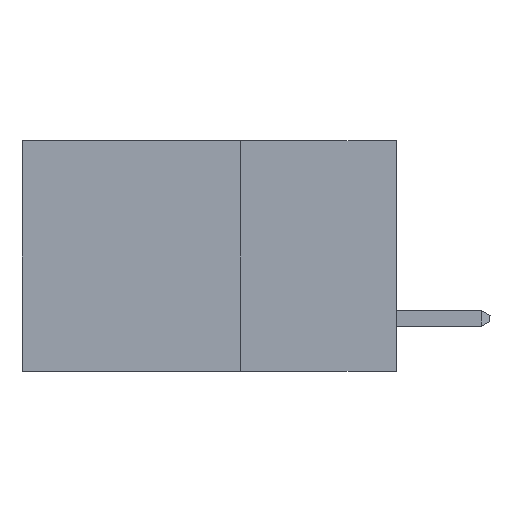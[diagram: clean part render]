
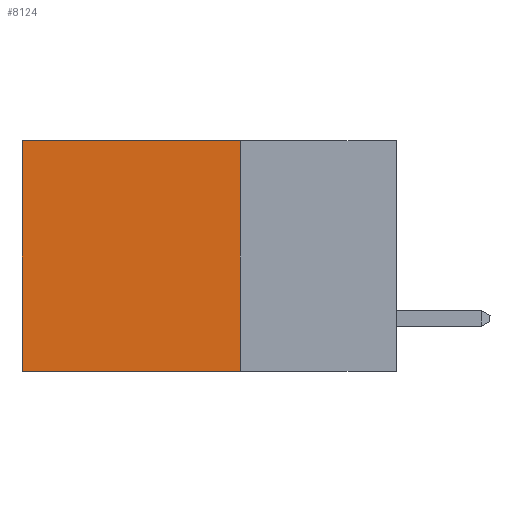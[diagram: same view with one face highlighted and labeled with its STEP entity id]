
A CAD part, left-side view. The second image highlights one B-rep face of the part: STEP entity #8124.
In plain terms, the highlighted planar face has unit normal (-1, 0, 0).
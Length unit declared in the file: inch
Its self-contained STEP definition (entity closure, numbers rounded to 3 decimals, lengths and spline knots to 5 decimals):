
#63 = VERTEX_POINT ( 'NONE', #6764 ) ;
#292 = DIRECTION ( 'NONE',  ( 0., 0., -1. ) ) ;
#690 = CARTESIAN_POINT ( 'NONE',  ( 0.2615, 0.25, -0.37 ) ) ;
#862 = VECTOR ( 'NONE', #292, 39.37008 ) ;
#1354 = CARTESIAN_POINT ( 'NONE',  ( 0.2615, 0.25, -0.37 ) ) ;
#1498 = DIRECTION ( 'NONE',  ( 0., 0., -1. ) ) ;
#1545 = FACE_OUTER_BOUND ( 'NONE', #8074, .T. ) ;
#1760 = ORIENTED_EDGE ( 'NONE', *, *, #3290, .F. ) ;
#1971 = LINE ( 'NONE', #5686, #862 ) ;
#2251 = DIRECTION ( 'NONE',  ( 1., 0., 0. ) ) ;
#2774 = EDGE_CURVE ( 'NONE', #63, #3135, #9484, .T. ) ;
#2840 = PLANE ( 'NONE',  #4221 ) ;
#3135 = VERTEX_POINT ( 'NONE', #9523 ) ;
#3290 = EDGE_CURVE ( 'NONE', #9681, #4045, #6729, .T. ) ;
#3715 = CARTESIAN_POINT ( 'NONE',  ( 0.2615, 0.6, -0.37 ) ) ;
#4045 = VERTEX_POINT ( 'NONE', #3715 ) ;
#4221 = AXIS2_PLACEMENT_3D ( 'NONE', #1354, #2251, #1498 ) ;
#4365 = VECTOR ( 'NONE', #9717, 39.37008 ) ;
#4622 = VECTOR ( 'NONE', #8279, 39.37008 ) ;
#4919 = EDGE_CURVE ( 'NONE', #3135, #4045, #1971, .T. ) ;
#5328 = LINE ( 'NONE', #8224, #4365 ) ;
#5660 = ORIENTED_EDGE ( 'NONE', *, *, #7139, .F. ) ;
#5686 = CARTESIAN_POINT ( 'NONE',  ( 0.2615, 0.6, -0.37 ) ) ;
#6640 = ORIENTED_EDGE ( 'NONE', *, *, #4919, .T. ) ;
#6729 = LINE ( 'NONE', #690, #4622 ) ;
#6764 = CARTESIAN_POINT ( 'NONE',  ( 0.2615, 0.25, 0. ) ) ;
#7139 = EDGE_CURVE ( 'NONE', #63, #9681, #5328, .T. ) ;
#7355 = CARTESIAN_POINT ( 'NONE',  ( 0.2615, 0.25, 0. ) ) ;
#7368 = VECTOR ( 'NONE', #8041, 39.37008 ) ;
#8041 = DIRECTION ( 'NONE',  ( 0., 1., 0. ) ) ;
#8074 = EDGE_LOOP ( 'NONE', ( #6640, #1760, #5660, #9621 ) ) ;
#8124 = ADVANCED_FACE ( 'NONE', ( #1545 ), #2840, .F. ) ;
#8224 = CARTESIAN_POINT ( 'NONE',  ( 0.2615, 0.25, -0.37 ) ) ;
#8253 = CARTESIAN_POINT ( 'NONE',  ( 0.2615, 0.25, -0.37 ) ) ;
#8279 = DIRECTION ( 'NONE',  ( 0., 1., 0. ) ) ;
#9484 = LINE ( 'NONE', #7355, #7368 ) ;
#9523 = CARTESIAN_POINT ( 'NONE',  ( 0.2615, 0.6, 0. ) ) ;
#9621 = ORIENTED_EDGE ( 'NONE', *, *, #2774, .T. ) ;
#9681 = VERTEX_POINT ( 'NONE', #8253 ) ;
#9717 = DIRECTION ( 'NONE',  ( 0., 0., -1. ) ) ;
